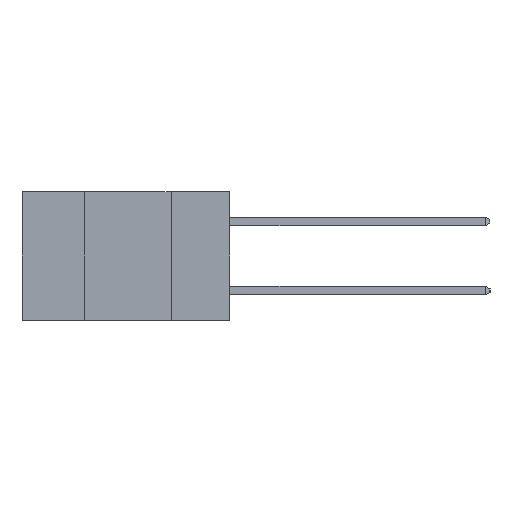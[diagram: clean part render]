
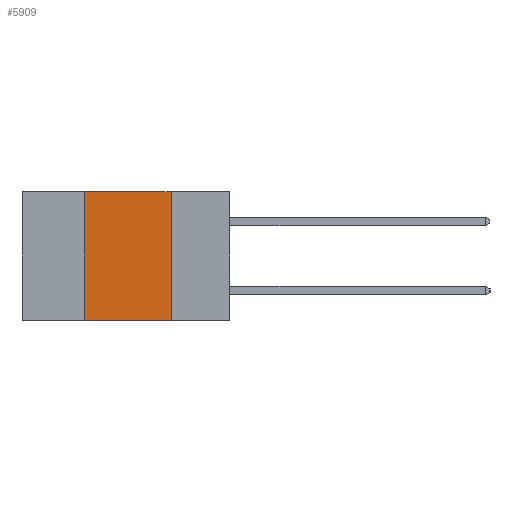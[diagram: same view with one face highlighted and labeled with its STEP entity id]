
A CAD part, left-side view. The second image highlights one B-rep face of the part: STEP entity #5909.
In plain terms, the highlighted planar face has unit normal (-1, 0, 0).
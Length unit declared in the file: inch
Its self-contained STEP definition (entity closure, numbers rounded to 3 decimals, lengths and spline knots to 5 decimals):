
#214 = LINE ( 'NONE', #2945, #14195 ) ;
#380 = EDGE_CURVE ( 'NONE', #6232, #2784, #1143, .T. ) ;
#550 = EDGE_LOOP ( 'NONE', ( #14160, #8558, #12472, #8921 ) ) ;
#1056 = EDGE_CURVE ( 'NONE', #7658, #3125, #10204, .T. ) ;
#1143 = LINE ( 'NONE', #12507, #7409 ) ;
#1169 = EDGE_CURVE ( 'NONE', #2784, #7658, #214, .T. ) ;
#1673 = DIRECTION ( 'NONE',  ( 0., 0., -1. ) ) ;
#1732 = DIRECTION ( 'NONE',  ( 1., 0., 0. ) ) ;
#1819 = PLANE ( 'NONE',  #3916 ) ;
#2784 = VERTEX_POINT ( 'NONE', #12290 ) ;
#2851 = CARTESIAN_POINT ( 'NONE',  ( 0., 0.17, -0.37 ) ) ;
#2864 = CARTESIAN_POINT ( 'NONE',  ( 0., 0.6, 0. ) ) ;
#2945 = CARTESIAN_POINT ( 'NONE',  ( 0., 0.6, 0. ) ) ;
#2992 = DIRECTION ( 'NONE',  ( 0., -1., 0. ) ) ;
#3125 = VERTEX_POINT ( 'NONE', #2851 ) ;
#3916 = AXIS2_PLACEMENT_3D ( 'NONE', #2864, #1732, #1673 ) ;
#4010 = LINE ( 'NONE', #10753, #12579 ) ;
#4408 = DIRECTION ( 'NONE',  ( 0., 0., -1. ) ) ;
#4440 = CARTESIAN_POINT ( 'NONE',  ( 0., 0.17, -0.37 ) ) ;
#5909 = ADVANCED_FACE ( 'NONE', ( #10456 ), #1819, .F. ) ;
#6232 = VERTEX_POINT ( 'NONE', #7931 ) ;
#7196 = VECTOR ( 'NONE', #4408, 39.37008 ) ;
#7409 = VECTOR ( 'NONE', #12418, 39.37008 ) ;
#7658 = VERTEX_POINT ( 'NONE', #8485 ) ;
#7931 = CARTESIAN_POINT ( 'NONE',  ( 0., 0.42, -0.37 ) ) ;
#8485 = CARTESIAN_POINT ( 'NONE',  ( 0., 0.17, 0. ) ) ;
#8558 = ORIENTED_EDGE ( 'NONE', *, *, #1169, .F. ) ;
#8921 = ORIENTED_EDGE ( 'NONE', *, *, #10417, .T. ) ;
#10204 = LINE ( 'NONE', #4440, #7196 ) ;
#10417 = EDGE_CURVE ( 'NONE', #6232, #3125, #4010, .T. ) ;
#10456 = FACE_OUTER_BOUND ( 'NONE', #550, .T. ) ;
#10753 = CARTESIAN_POINT ( 'NONE',  ( 0., 0.6, -0.37 ) ) ;
#10983 = DIRECTION ( 'NONE',  ( 0., -1., 0. ) ) ;
#12290 = CARTESIAN_POINT ( 'NONE',  ( 0., 0.42, 0. ) ) ;
#12418 = DIRECTION ( 'NONE',  ( 0., 0., 1. ) ) ;
#12472 = ORIENTED_EDGE ( 'NONE', *, *, #380, .F. ) ;
#12507 = CARTESIAN_POINT ( 'NONE',  ( 0., 0.42, -0.37 ) ) ;
#12579 = VECTOR ( 'NONE', #10983, 39.37008 ) ;
#14160 = ORIENTED_EDGE ( 'NONE', *, *, #1056, .F. ) ;
#14195 = VECTOR ( 'NONE', #2992, 39.37008 ) ;
